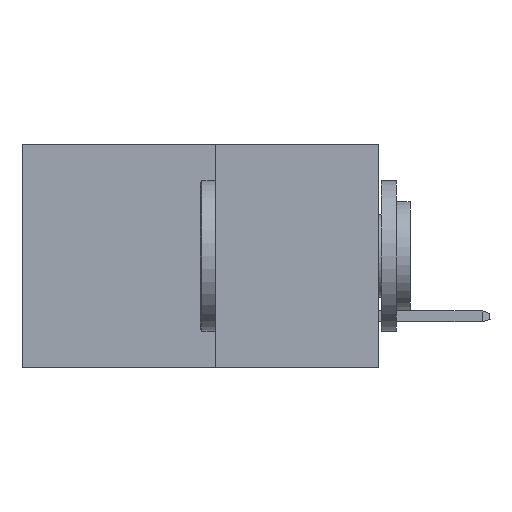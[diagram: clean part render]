
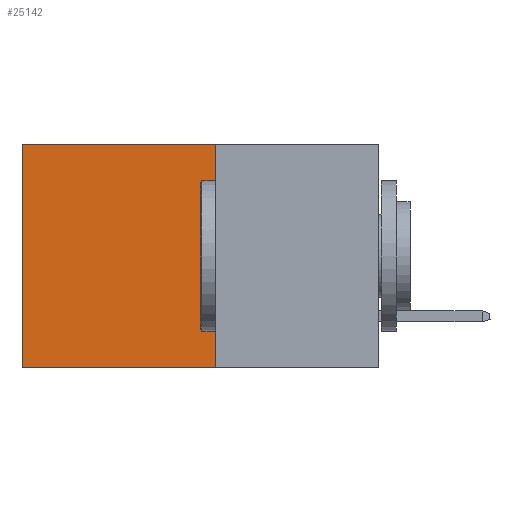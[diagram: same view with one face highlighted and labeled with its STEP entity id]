
A CAD part, left-side view. The second image highlights one B-rep face of the part: STEP entity #25142.
In plain terms, the highlighted planar face has unit normal (-1, 0, 0).
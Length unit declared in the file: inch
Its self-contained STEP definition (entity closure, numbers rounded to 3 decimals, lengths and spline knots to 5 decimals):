
#1833 = LINE ( 'NONE', #29888, #28977 ) ;
#4110 = AXIS2_PLACEMENT_3D ( 'NONE', #23263, #28564, #12930 ) ;
#5205 = VERTEX_POINT ( 'NONE', #13368 ) ;
#6326 = VERTEX_POINT ( 'NONE', #14805 ) ;
#6793 = EDGE_CURVE ( 'NONE', #6326, #14133, #1833, .T. ) ;
#7108 = CARTESIAN_POINT ( 'NONE',  ( 0.277, 0.27, -0.37 ) ) ;
#8839 = ORIENTED_EDGE ( 'NONE', *, *, #6793, .T. ) ;
#8900 = LINE ( 'NONE', #7108, #22934 ) ;
#9950 = CARTESIAN_POINT ( 'NONE',  ( 0.277, 0.59, -0.37 ) ) ;
#9998 = FACE_OUTER_BOUND ( 'NONE', #21505, .T. ) ;
#11190 = EDGE_CURVE ( 'NONE', #5205, #30090, #13041, .T. ) ;
#12541 = CARTESIAN_POINT ( 'NONE',  ( 0.277, 0.59, 0. ) ) ;
#12930 = DIRECTION ( 'NONE',  ( 0., 0., -1. ) ) ;
#13041 = LINE ( 'NONE', #13874, #14673 ) ;
#13368 = CARTESIAN_POINT ( 'NONE',  ( 0.277, 0.27, -0.37 ) ) ;
#13874 = CARTESIAN_POINT ( 'NONE',  ( 0.277, 0.27, -0.37 ) ) ;
#14133 = VERTEX_POINT ( 'NONE', #12541 ) ;
#14673 = VECTOR ( 'NONE', #32098, 39.37008 ) ;
#14805 = CARTESIAN_POINT ( 'NONE',  ( 0.277, 0.27, 0. ) ) ;
#15261 = DIRECTION ( 'NONE',  ( 0., 0., -1. ) ) ;
#15829 = CARTESIAN_POINT ( 'NONE',  ( 0.277, 0.59, -0.37 ) ) ;
#19910 = ORIENTED_EDGE ( 'NONE', *, *, #23252, .F. ) ;
#20702 = PLANE ( 'NONE',  #4110 ) ;
#21374 = VECTOR ( 'NONE', #15261, 39.37008 ) ;
#21505 = EDGE_LOOP ( 'NONE', ( #23006, #33519, #19910, #8839 ) ) ;
#22934 = VECTOR ( 'NONE', #25522, 39.37008 ) ;
#23006 = ORIENTED_EDGE ( 'NONE', *, *, #27791, .T. ) ;
#23252 = EDGE_CURVE ( 'NONE', #6326, #5205, #8900, .T. ) ;
#23263 = CARTESIAN_POINT ( 'NONE',  ( 0.277, 0.27, -0.37 ) ) ;
#25142 = ADVANCED_FACE ( 'NONE', ( #9998 ), #20702, .F. ) ;
#25522 = DIRECTION ( 'NONE',  ( 0., 0., -1. ) ) ;
#27791 = EDGE_CURVE ( 'NONE', #14133, #30090, #28291, .T. ) ;
#28291 = LINE ( 'NONE', #9950, #21374 ) ;
#28564 = DIRECTION ( 'NONE',  ( 1., 0., 0. ) ) ;
#28977 = VECTOR ( 'NONE', #29436, 39.37008 ) ;
#29436 = DIRECTION ( 'NONE',  ( 0., 1., 0. ) ) ;
#29888 = CARTESIAN_POINT ( 'NONE',  ( 0.277, 0.27, 0. ) ) ;
#30090 = VERTEX_POINT ( 'NONE', #15829 ) ;
#32098 = DIRECTION ( 'NONE',  ( 0., 1., 0. ) ) ;
#33519 = ORIENTED_EDGE ( 'NONE', *, *, #11190, .F. ) ;
